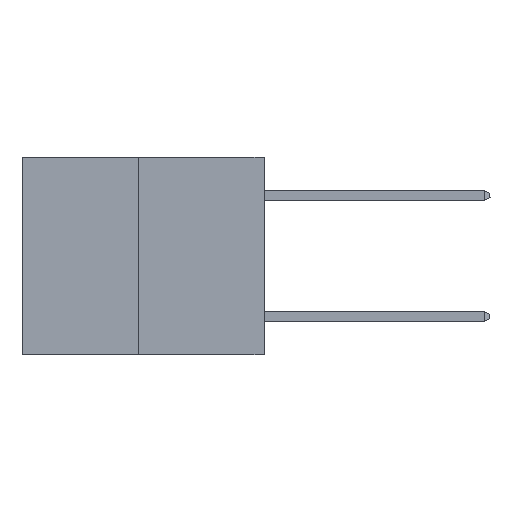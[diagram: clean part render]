
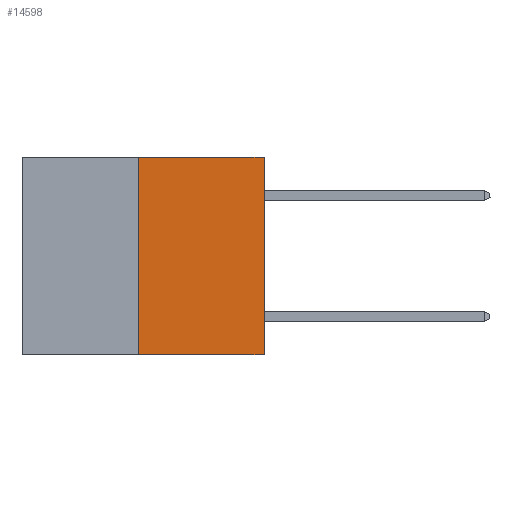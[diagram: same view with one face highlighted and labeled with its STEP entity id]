
A CAD part, left-side view. The second image highlights one B-rep face of the part: STEP entity #14598.
In plain terms, the highlighted planar face has unit normal (-1, 0, 0).
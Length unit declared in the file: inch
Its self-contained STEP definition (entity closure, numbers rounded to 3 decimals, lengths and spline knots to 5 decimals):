
#335 = AXIS2_PLACEMENT_3D ( 'NONE', #712, #14290, #28424 ) ;
#610 = VECTOR ( 'NONE', #25945, 39.37008 ) ;
#664 = CARTESIAN_POINT ( 'NONE',  ( 0., 0., 0. ) ) ;
#712 = CARTESIAN_POINT ( 'NONE',  ( 0., 0.6, 0. ) ) ;
#1085 = DIRECTION ( 'NONE',  ( 0., -1., 0. ) ) ;
#2436 = DIRECTION ( 'NONE',  ( 0., 0., 1. ) ) ;
#3224 = VERTEX_POINT ( 'NONE', #664 ) ;
#3615 = LINE ( 'NONE', #14672, #23139 ) ;
#5191 = LINE ( 'NONE', #27368, #28970 ) ;
#8962 = ORIENTED_EDGE ( 'NONE', *, *, #29026, .T. ) ;
#9649 = EDGE_CURVE ( 'NONE', #25772, #3224, #5191, .T. ) ;
#12722 = ORIENTED_EDGE ( 'NONE', *, *, #27252, .F. ) ;
#14290 = DIRECTION ( 'NONE',  ( 1., 0., 0. ) ) ;
#14578 = CARTESIAN_POINT ( 'NONE',  ( 0., 0., -0.49 ) ) ;
#14598 = ADVANCED_FACE ( 'NONE', ( #16275 ), #16539, .F. ) ;
#14672 = CARTESIAN_POINT ( 'NONE',  ( 0., 0.6, 0. ) ) ;
#16275 = FACE_OUTER_BOUND ( 'NONE', #25662, .T. ) ;
#16355 = ORIENTED_EDGE ( 'NONE', *, *, #26912, .F. ) ;
#16539 = PLANE ( 'NONE',  #335 ) ;
#17323 = VECTOR ( 'NONE', #2436, 39.37008 ) ;
#18011 = VERTEX_POINT ( 'NONE', #26267 ) ;
#18036 = LINE ( 'NONE', #27635, #17323 ) ;
#22545 = CARTESIAN_POINT ( 'NONE',  ( 0., 0.312, -0.49 ) ) ;
#23139 = VECTOR ( 'NONE', #1085, 39.37008 ) ;
#25662 = EDGE_LOOP ( 'NONE', ( #16355, #8962, #26898, #12722 ) ) ;
#25772 = VERTEX_POINT ( 'NONE', #14578 ) ;
#25945 = DIRECTION ( 'NONE',  ( 0., -1., 0. ) ) ;
#26267 = CARTESIAN_POINT ( 'NONE',  ( 0., 0.312, 0. ) ) ;
#26453 = VERTEX_POINT ( 'NONE', #22545 ) ;
#26898 = ORIENTED_EDGE ( 'NONE', *, *, #9649, .T. ) ;
#26912 = EDGE_CURVE ( 'NONE', #26453, #18011, #18036, .T. ) ;
#27252 = EDGE_CURVE ( 'NONE', #18011, #3224, #3615, .T. ) ;
#27368 = CARTESIAN_POINT ( 'NONE',  ( 0., 0., 0. ) ) ;
#27635 = CARTESIAN_POINT ( 'NONE',  ( 0., 0.312, -0.49 ) ) ;
#28246 = CARTESIAN_POINT ( 'NONE',  ( 0., 0.6, -0.49 ) ) ;
#28378 = LINE ( 'NONE', #28246, #610 ) ;
#28424 = DIRECTION ( 'NONE',  ( 0., 0., -1. ) ) ;
#28970 = VECTOR ( 'NONE', #29435, 39.37008 ) ;
#29026 = EDGE_CURVE ( 'NONE', #26453, #25772, #28378, .T. ) ;
#29435 = DIRECTION ( 'NONE',  ( 0., 0., 1. ) ) ;
